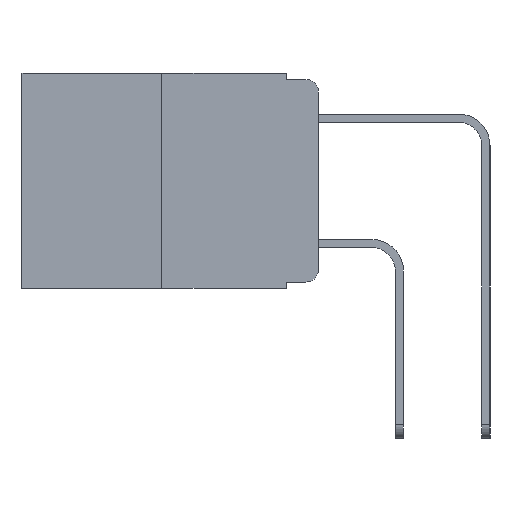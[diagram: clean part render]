
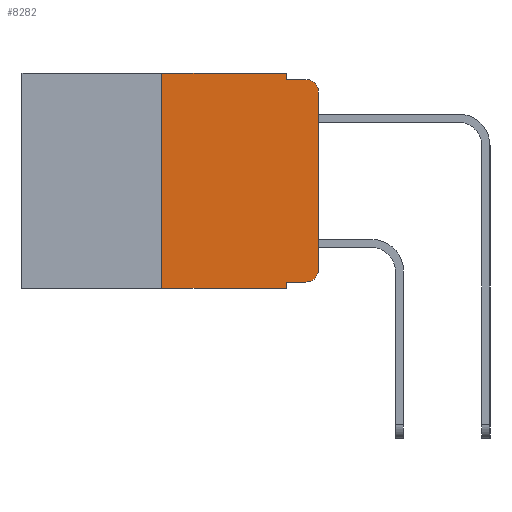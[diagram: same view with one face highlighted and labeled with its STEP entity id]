
A CAD part, left-side view. The second image highlights one B-rep face of the part: STEP entity #8282.
In plain terms, the highlighted planar face has unit normal (-1, 0, 0).
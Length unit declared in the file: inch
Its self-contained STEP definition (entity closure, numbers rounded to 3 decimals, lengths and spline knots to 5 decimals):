
#58 = VERTEX_POINT ( 'NONE', #258 ) ;
#61 = VERTEX_POINT ( 'NONE', #14269 ) ;
#258 = CARTESIAN_POINT ( 'NONE',  ( 0., 0.25, 0. ) ) ;
#281 = CARTESIAN_POINT ( 'NONE',  ( 0., 0.02, -0.03 ) ) ;
#528 = ORIENTED_EDGE ( 'NONE', *, *, #15696, .T. ) ;
#660 = VERTEX_POINT ( 'NONE', #17260 ) ;
#775 = LINE ( 'NONE', #18477, #4474 ) ;
#975 = ORIENTED_EDGE ( 'NONE', *, *, #14729, .T. ) ;
#1009 = VERTEX_POINT ( 'NONE', #17219 ) ;
#1244 = DIRECTION ( 'NONE',  ( 0., 0., -1. ) ) ;
#1555 = DIRECTION ( 'NONE',  ( 0., -1., 0. ) ) ;
#1618 = DIRECTION ( 'NONE',  ( -1., 0., 0. ) ) ;
#1905 = DIRECTION ( 'NONE',  ( 0., 0., -1. ) ) ;
#1984 = CARTESIAN_POINT ( 'NONE',  ( 0., 0.051, -0.343 ) ) ;
#2504 = VERTEX_POINT ( 'NONE', #15397 ) ;
#2677 = VECTOR ( 'NONE', #11877, 39.37008 ) ;
#2735 = VECTOR ( 'NONE', #15274, 39.37008 ) ;
#3219 = CARTESIAN_POINT ( 'NONE',  ( 0., 0., -0.313 ) ) ;
#3236 = VECTOR ( 'NONE', #1555, 39.37008 ) ;
#3814 = CARTESIAN_POINT ( 'NONE',  ( 0., 0.473, 0. ) ) ;
#3977 = CARTESIAN_POINT ( 'NONE',  ( 0., 0.051, -0.01 ) ) ;
#4474 = VECTOR ( 'NONE', #9595, 39.37008 ) ;
#5069 = CARTESIAN_POINT ( 'NONE',  ( 0., 0.051, 0. ) ) ;
#5536 = CARTESIAN_POINT ( 'NONE',  ( 0., 0.051, -0.333 ) ) ;
#6182 = VECTOR ( 'NONE', #12964, 39.37008 ) ;
#6287 = EDGE_CURVE ( 'NONE', #18570, #61, #15341, .T. ) ;
#6644 = DIRECTION ( 'NONE',  ( 0., 0., -1. ) ) ;
#7314 = EDGE_CURVE ( 'NONE', #1009, #61, #17361, .T. ) ;
#8282 = ADVANCED_FACE ( 'NONE', ( #11024 ), #14929, .F. ) ;
#8283 = VERTEX_POINT ( 'NONE', #8948 ) ;
#8565 = EDGE_CURVE ( 'NONE', #2504, #15518, #12200, .T. ) ;
#8770 = AXIS2_PLACEMENT_3D ( 'NONE', #281, #11171, #1905 ) ;
#8778 = CARTESIAN_POINT ( 'NONE',  ( 0., 0.25, 0. ) ) ;
#8948 = CARTESIAN_POINT ( 'NONE',  ( 0., 0.051, -0.333 ) ) ;
#9202 = CARTESIAN_POINT ( 'NONE',  ( 0., 0.473, -0.343 ) ) ;
#9257 = ORIENTED_EDGE ( 'NONE', *, *, #16688, .F. ) ;
#9298 = ORIENTED_EDGE ( 'NONE', *, *, #8565, .T. ) ;
#9339 = EDGE_CURVE ( 'NONE', #17986, #1009, #775, .T. ) ;
#9411 = ORIENTED_EDGE ( 'NONE', *, *, #18662, .F. ) ;
#9491 = EDGE_CURVE ( 'NONE', #58, #15043, #18109, .T. ) ;
#9510 = ORIENTED_EDGE ( 'NONE', *, *, #9491, .F. ) ;
#9595 = DIRECTION ( 'NONE',  ( 0., 0., 1. ) ) ;
#10524 = DIRECTION ( 'NONE',  ( 1., 0., 0. ) ) ;
#10637 = VECTOR ( 'NONE', #13194, 39.37008 ) ;
#10765 = VECTOR ( 'NONE', #15165, 39.37008 ) ;
#10873 = CARTESIAN_POINT ( 'NONE',  ( 0., 0.02, -0.313 ) ) ;
#10953 = ORIENTED_EDGE ( 'NONE', *, *, #9339, .T. ) ;
#11024 = FACE_OUTER_BOUND ( 'NONE', #16200, .T. ) ;
#11171 = DIRECTION ( 'NONE',  ( -1., 0., 0. ) ) ;
#11877 = DIRECTION ( 'NONE',  ( 0., 0., 1. ) ) ;
#12200 = LINE ( 'NONE', #9202, #10765 ) ;
#12400 = DIRECTION ( 'NONE',  ( 0., 0., -1. ) ) ;
#12571 = CIRCLE ( 'NONE', #12586, 0.02 ) ;
#12586 = AXIS2_PLACEMENT_3D ( 'NONE', #10873, #1618, #12400 ) ;
#12844 = ORIENTED_EDGE ( 'NONE', *, *, #6287, .F. ) ;
#12924 = ORIENTED_EDGE ( 'NONE', *, *, #19595, .F. ) ;
#12964 = DIRECTION ( 'NONE',  ( 0., -1., 0. ) ) ;
#12967 = LINE ( 'NONE', #5069, #16859 ) ;
#13194 = DIRECTION ( 'NONE',  ( 0., -1., 0. ) ) ;
#13814 = CARTESIAN_POINT ( 'NONE',  ( 0., 0.051, 0. ) ) ;
#14269 = CARTESIAN_POINT ( 'NONE',  ( 0., 0.02, -0.01 ) ) ;
#14553 = CARTESIAN_POINT ( 'NONE',  ( 0., 0.051, 0. ) ) ;
#14582 = LINE ( 'NONE', #5536, #10637 ) ;
#14729 = EDGE_CURVE ( 'NONE', #660, #17986, #12571, .T. ) ;
#14821 = LINE ( 'NONE', #8778, #2677 ) ;
#14826 = ORIENTED_EDGE ( 'NONE', *, *, #7314, .T. ) ;
#14929 = PLANE ( 'NONE',  #19580 ) ;
#15043 = VERTEX_POINT ( 'NONE', #14553 ) ;
#15165 = DIRECTION ( 'NONE',  ( 0., -1., 0. ) ) ;
#15274 = DIRECTION ( 'NONE',  ( 0., 0., -1. ) ) ;
#15341 = LINE ( 'NONE', #18181, #3236 ) ;
#15397 = CARTESIAN_POINT ( 'NONE',  ( 0., 0.25, -0.343 ) ) ;
#15518 = VERTEX_POINT ( 'NONE', #1984 ) ;
#15696 = EDGE_CURVE ( 'NONE', #8283, #660, #14582, .T. ) ;
#16200 = EDGE_LOOP ( 'NONE', ( #10953, #14826, #12844, #12924, #9510, #9411, #9298, #9257, #528, #975 ) ) ;
#16688 = EDGE_CURVE ( 'NONE', #8283, #15518, #18324, .T. ) ;
#16859 = VECTOR ( 'NONE', #6644, 39.37008 ) ;
#17219 = CARTESIAN_POINT ( 'NONE',  ( 0., 0., -0.03 ) ) ;
#17260 = CARTESIAN_POINT ( 'NONE',  ( 0., 0.02, -0.333 ) ) ;
#17361 = CIRCLE ( 'NONE', #8770, 0.02 ) ;
#17986 = VERTEX_POINT ( 'NONE', #3219 ) ;
#18109 = LINE ( 'NONE', #3814, #6182 ) ;
#18181 = CARTESIAN_POINT ( 'NONE',  ( 0., 0.051, -0.01 ) ) ;
#18324 = LINE ( 'NONE', #13814, #2735 ) ;
#18477 = CARTESIAN_POINT ( 'NONE',  ( 0., 0., 0. ) ) ;
#18570 = VERTEX_POINT ( 'NONE', #3977 ) ;
#18662 = EDGE_CURVE ( 'NONE', #2504, #58, #14821, .T. ) ;
#19325 = CARTESIAN_POINT ( 'NONE',  ( 0., 0.473, 0. ) ) ;
#19580 = AXIS2_PLACEMENT_3D ( 'NONE', #19325, #10524, #1244 ) ;
#19595 = EDGE_CURVE ( 'NONE', #15043, #18570, #12967, .T. ) ;
